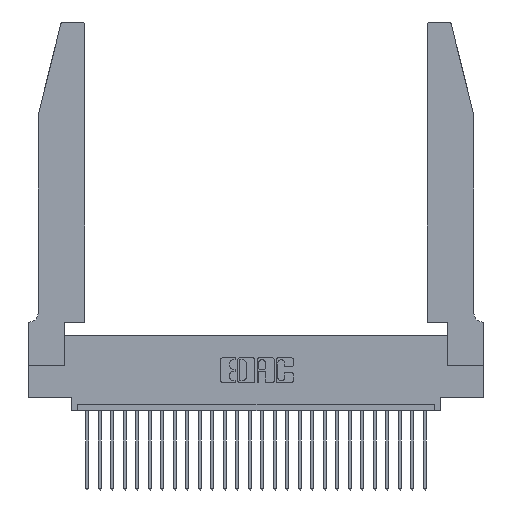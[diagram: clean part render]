
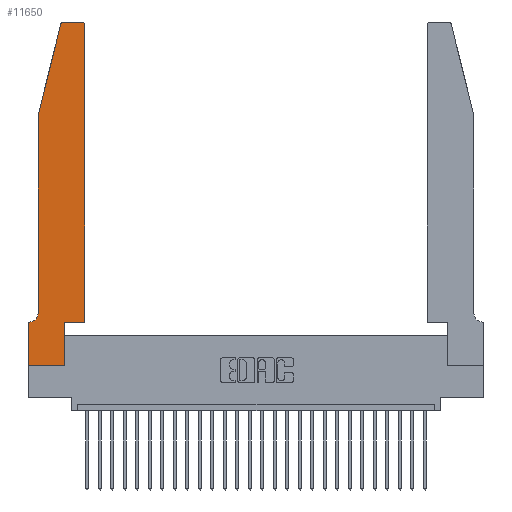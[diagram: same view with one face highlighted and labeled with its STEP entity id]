
A CAD part, top view. The second image highlights one B-rep face of the part: STEP entity #11650.
In plain terms, the highlighted planar face has unit normal (0, 0, 1).
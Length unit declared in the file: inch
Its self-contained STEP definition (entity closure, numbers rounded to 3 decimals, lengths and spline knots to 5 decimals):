
#374 = DIRECTION ( 'NONE',  ( 1., 0., 0. ) ) ;
#772 = CARTESIAN_POINT ( 'NONE',  ( 0., 0., 0.37 ) ) ;
#977 = VECTOR ( 'NONE', #27153, 39.37008 ) ;
#1113 = EDGE_CURVE ( 'NONE', #27810, #25946, #8180, .T. ) ;
#3008 = ORIENTED_EDGE ( 'NONE', *, *, #1113, .T. ) ;
#3283 = CARTESIAN_POINT ( 'NONE',  ( 0.25487, 2.72718, 0.37 ) ) ;
#3616 = CARTESIAN_POINT ( 'NONE',  ( 0.0055, 0.42, 0.37 ) ) ;
#3797 = EDGE_CURVE ( 'NONE', #10068, #24101, #14407, .T. ) ;
#3799 = VECTOR ( 'NONE', #5652, 39.37008 ) ;
#3877 = EDGE_CURVE ( 'NONE', #7825, #6305, #16786, .T. ) ;
#4088 = CIRCLE ( 'NONE', #20732, 0.03 ) ;
#4143 = ORIENTED_EDGE ( 'NONE', *, *, #18256, .T. ) ;
#4221 = CARTESIAN_POINT ( 'NONE',  ( 0.0755, 2., 0.37 ) ) ;
#4458 = EDGE_CURVE ( 'NONE', #9141, #10068, #10382, .T. ) ;
#4695 = CARTESIAN_POINT ( 'NONE',  ( 0.4505, 0.35, 0.37 ) ) ;
#4964 = ORIENTED_EDGE ( 'NONE', *, *, #6964, .T. ) ;
#4974 = CARTESIAN_POINT ( 'NONE',  ( 0., 0., 0.37 ) ) ;
#5245 = LINE ( 'NONE', #4695, #27396 ) ;
#5381 = AXIS2_PLACEMENT_3D ( 'NONE', #3616, #18312, #18683 ) ;
#5385 = EDGE_CURVE ( 'NONE', #16863, #7825, #12980, .T. ) ;
#5612 = VECTOR ( 'NONE', #20713, 39.37008 ) ;
#5652 = DIRECTION ( 'NONE',  ( 1., 0., 0. ) ) ;
#5711 = DIRECTION ( 'NONE',  ( 0., 0., 1. ) ) ;
#5961 = EDGE_CURVE ( 'NONE', #13286, #27810, #26062, .T. ) ;
#6194 = VERTEX_POINT ( 'NONE', #7562 ) ;
#6305 = VERTEX_POINT ( 'NONE', #15122 ) ;
#6742 = LINE ( 'NONE', #22874, #977 ) ;
#6964 = EDGE_CURVE ( 'NONE', #8910, #16863, #22327, .T. ) ;
#7266 = VERTEX_POINT ( 'NONE', #3283 ) ;
#7435 = ORIENTED_EDGE ( 'NONE', *, *, #8695, .T. ) ;
#7562 = CARTESIAN_POINT ( 'NONE',  ( 0., 0.35, 0.37 ) ) ;
#7598 = DIRECTION ( 'NONE',  ( 1., 0., 0. ) ) ;
#7786 = CARTESIAN_POINT ( 'NONE',  ( 0.4205, 2.75, 0.37 ) ) ;
#7825 = VERTEX_POINT ( 'NONE', #17137 ) ;
#8180 = CIRCLE ( 'NONE', #5381, 0.07 ) ;
#8695 = EDGE_CURVE ( 'NONE', #7266, #13286, #6742, .T. ) ;
#8910 = VERTEX_POINT ( 'NONE', #772 ) ;
#8963 = CARTESIAN_POINT ( 'NONE',  ( 0.0755, 2., 0.37 ) ) ;
#9141 = VERTEX_POINT ( 'NONE', #19842 ) ;
#9273 = DIRECTION ( 'NONE',  ( 0., -1., 0. ) ) ;
#9523 = LINE ( 'NONE', #25491, #23997 ) ;
#9697 = VECTOR ( 'NONE', #10546, 39.37008 ) ;
#10067 = EDGE_CURVE ( 'NONE', #24101, #7266, #4088, .T. ) ;
#10068 = VERTEX_POINT ( 'NONE', #7786 ) ;
#10076 = DIRECTION ( 'NONE',  ( 1., 0., 0. ) ) ;
#10162 = DIRECTION ( 'NONE',  ( 1., 0., 0. ) ) ;
#10382 = CIRCLE ( 'NONE', #26477, 0.03 ) ;
#10546 = DIRECTION ( 'NONE',  ( -1., 0., 0. ) ) ;
#11344 = DIRECTION ( 'NONE',  ( 0., 1., 0. ) ) ;
#11650 = ADVANCED_FACE ( 'NONE', ( #26499 ), #24341, .T. ) ;
#12379 = VECTOR ( 'NONE', #10076, 39.37008 ) ;
#12980 = LINE ( 'NONE', #14108, #5612 ) ;
#13100 = DIRECTION ( 'NONE',  ( 0., 0., 1. ) ) ;
#13286 = VERTEX_POINT ( 'NONE', #8963 ) ;
#13523 = AXIS2_PLACEMENT_3D ( 'NONE', #26670, #14181, #10162 ) ;
#13954 = VECTOR ( 'NONE', #26084, 39.37008 ) ;
#14108 = CARTESIAN_POINT ( 'NONE',  ( 0.2865, 0.35, 0.37 ) ) ;
#14181 = DIRECTION ( 'NONE',  ( 0., 0., 1. ) ) ;
#14407 = LINE ( 'NONE', #14832, #9697 ) ;
#14832 = CARTESIAN_POINT ( 'NONE',  ( 0.2605, 2.75, 0.37 ) ) ;
#14935 = ORIENTED_EDGE ( 'NONE', *, *, #4458, .T. ) ;
#15122 = CARTESIAN_POINT ( 'NONE',  ( 0.4505, 0.35, 0.37 ) ) ;
#15566 = ORIENTED_EDGE ( 'NONE', *, *, #5385, .T. ) ;
#15621 = ORIENTED_EDGE ( 'NONE', *, *, #25155, .T. ) ;
#15736 = CARTESIAN_POINT ( 'NONE',  ( 0.284, 2.75, 0.37 ) ) ;
#16786 = LINE ( 'NONE', #22952, #12379 ) ;
#16863 = VERTEX_POINT ( 'NONE', #18789 ) ;
#17137 = CARTESIAN_POINT ( 'NONE',  ( 0.2865, 0.35, 0.37 ) ) ;
#17305 = ORIENTED_EDGE ( 'NONE', *, *, #26205, .T. ) ;
#17980 = CARTESIAN_POINT ( 'NONE',  ( 0.0055, 0.35, 0.37 ) ) ;
#18256 = EDGE_CURVE ( 'NONE', #6194, #8910, #25517, .T. ) ;
#18312 = DIRECTION ( 'NONE',  ( 0., 0., -1. ) ) ;
#18439 = ORIENTED_EDGE ( 'NONE', *, *, #5961, .T. ) ;
#18683 = DIRECTION ( 'NONE',  ( -1., 0., 0. ) ) ;
#18789 = CARTESIAN_POINT ( 'NONE',  ( 0.2865, 0., 0.37 ) ) ;
#18997 = EDGE_LOOP ( 'NONE', ( #26651, #23830, #7435, #18439, #3008, #17305, #4143, #4964, #15566, #25833, #15621, #14935 ) ) ;
#19842 = CARTESIAN_POINT ( 'NONE',  ( 0.4505, 2.72, 0.37 ) ) ;
#20713 = DIRECTION ( 'NONE',  ( 0., 1., 0. ) ) ;
#20732 = AXIS2_PLACEMENT_3D ( 'NONE', #22634, #5711, #7598 ) ;
#20815 = VECTOR ( 'NONE', #9273, 39.37008 ) ;
#21709 = CARTESIAN_POINT ( 'NONE',  ( 0.4205, 2.72, 0.37 ) ) ;
#22327 = LINE ( 'NONE', #27233, #3799 ) ;
#22634 = CARTESIAN_POINT ( 'NONE',  ( 0.284, 2.72, 0.37 ) ) ;
#22874 = CARTESIAN_POINT ( 'NONE',  ( 0.0755, 2., 0.37 ) ) ;
#22952 = CARTESIAN_POINT ( 'NONE',  ( 0.4505, 0.35, 0.37 ) ) ;
#23830 = ORIENTED_EDGE ( 'NONE', *, *, #10067, .T. ) ;
#23997 = VECTOR ( 'NONE', #27618, 39.37008 ) ;
#24101 = VERTEX_POINT ( 'NONE', #15736 ) ;
#24341 = PLANE ( 'NONE',  #13523 ) ;
#25020 = CARTESIAN_POINT ( 'NONE',  ( 0.0755, 0.42, 0.37 ) ) ;
#25155 = EDGE_CURVE ( 'NONE', #6305, #9141, #5245, .T. ) ;
#25491 = CARTESIAN_POINT ( 'NONE',  ( 0.0755, 0.35, 0.37 ) ) ;
#25517 = LINE ( 'NONE', #4974, #20815 ) ;
#25833 = ORIENTED_EDGE ( 'NONE', *, *, #3877, .T. ) ;
#25946 = VERTEX_POINT ( 'NONE', #17980 ) ;
#26062 = LINE ( 'NONE', #4221, #13954 ) ;
#26084 = DIRECTION ( 'NONE',  ( 0., -1., 0. ) ) ;
#26205 = EDGE_CURVE ( 'NONE', #25946, #6194, #9523, .T. ) ;
#26477 = AXIS2_PLACEMENT_3D ( 'NONE', #21709, #13100, #374 ) ;
#26499 = FACE_OUTER_BOUND ( 'NONE', #18997, .T. ) ;
#26651 = ORIENTED_EDGE ( 'NONE', *, *, #3797, .T. ) ;
#26670 = CARTESIAN_POINT ( 'NONE',  ( 0., 0.35, 0.37 ) ) ;
#27153 = DIRECTION ( 'NONE',  ( -0.239, -0.971, 0. ) ) ;
#27233 = CARTESIAN_POINT ( 'NONE',  ( 0., 0., 0.37 ) ) ;
#27396 = VECTOR ( 'NONE', #11344, 39.37008 ) ;
#27618 = DIRECTION ( 'NONE',  ( -1., 0., 0. ) ) ;
#27810 = VERTEX_POINT ( 'NONE', #25020 ) ;
